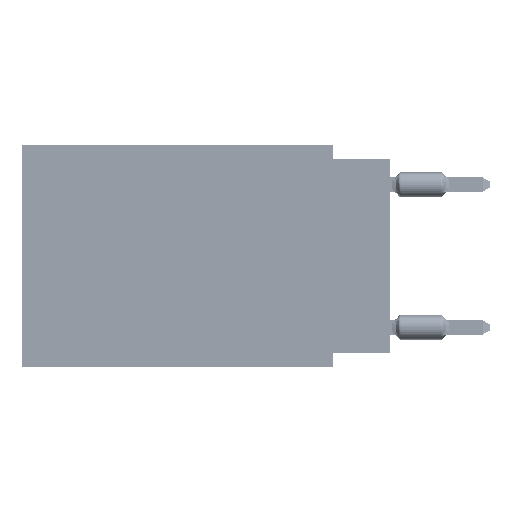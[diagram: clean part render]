
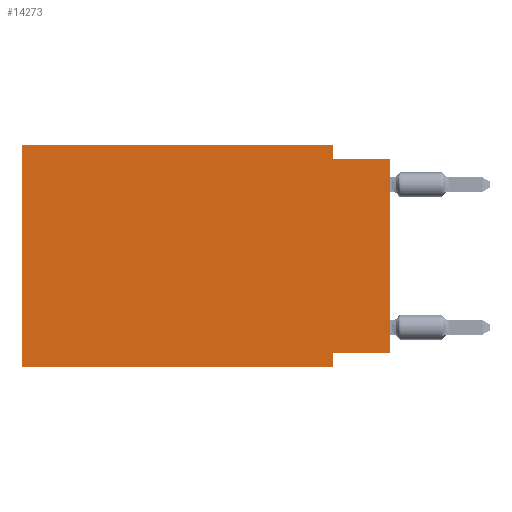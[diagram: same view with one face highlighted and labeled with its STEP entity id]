
A CAD part, left-side view. The second image highlights one B-rep face of the part: STEP entity #14273.
In plain terms, the highlighted planar face has unit normal (-1, 0, 0).
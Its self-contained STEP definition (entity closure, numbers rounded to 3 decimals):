
#194 = EDGE_CURVE ( 'NONE', #3781, #33344, #15759, .T. ) ;
#601 = CARTESIAN_POINT ( 'NONE',  ( 0., 0., -9.271 ) ) ;
#1645 = DIRECTION ( 'NONE',  ( 0., 0., 1. ) ) ;
#1699 = LINE ( 'NONE', #14349, #16346 ) ;
#2934 = ORIENTED_EDGE ( 'NONE', *, *, #26438, .F. ) ;
#3781 = VERTEX_POINT ( 'NONE', #601 ) ;
#3854 = VECTOR ( 'NONE', #1645, 1000. ) ;
#4674 = CARTESIAN_POINT ( 'NONE',  ( 0., 0., -0.635 ) ) ;
#5624 = VERTEX_POINT ( 'NONE', #8807 ) ;
#5972 = DIRECTION ( 'NONE',  ( 0., -1., 0. ) ) ;
#7640 = CARTESIAN_POINT ( 'NONE',  ( 0., 0., 0. ) ) ;
#8581 = DIRECTION ( 'NONE',  ( 0., -1., 0. ) ) ;
#8807 = CARTESIAN_POINT ( 'NONE',  ( 0., 2.54, -0.635 ) ) ;
#9232 = ORIENTED_EDGE ( 'NONE', *, *, #44847, .F. ) ;
#9246 = CARTESIAN_POINT ( 'NONE',  ( 0., 16.383, 0. ) ) ;
#10726 = DIRECTION ( 'NONE',  ( 0., -1., 0. ) ) ;
#11230 = CARTESIAN_POINT ( 'NONE',  ( 0., 2.54, 0. ) ) ;
#11405 = EDGE_CURVE ( 'NONE', #27333, #56095, #11659, .T. ) ;
#11659 = LINE ( 'NONE', #47135, #54206 ) ;
#13464 = EDGE_CURVE ( 'NONE', #56095, #5624, #46716, .T. ) ;
#14273 = ADVANCED_FACE ( 'NONE', ( #47456 ), #15294, .F. ) ;
#14349 = CARTESIAN_POINT ( 'NONE',  ( 0., 16.383, -9.906 ) ) ;
#14377 = CARTESIAN_POINT ( 'NONE',  ( 0., 2.54, -9.906 ) ) ;
#15294 = PLANE ( 'NONE',  #59230 ) ;
#15759 = LINE ( 'NONE', #7640, #3854 ) ;
#16346 = VECTOR ( 'NONE', #10726, 1000. ) ;
#16832 = ORIENTED_EDGE ( 'NONE', *, *, #58958, .F. ) ;
#17105 = ORIENTED_EDGE ( 'NONE', *, *, #44590, .T. ) ;
#19935 = EDGE_CURVE ( 'NONE', #44087, #50458, #32715, .T. ) ;
#23075 = DIRECTION ( 'NONE',  ( 0., 0., 1. ) ) ;
#23708 = CARTESIAN_POINT ( 'NONE',  ( 0., 0., -9.271 ) ) ;
#26438 = EDGE_CURVE ( 'NONE', #3781, #44087, #45647, .T. ) ;
#27333 = VERTEX_POINT ( 'NONE', #48832 ) ;
#27657 = CARTESIAN_POINT ( 'NONE',  ( 0., 2.54, -9.271 ) ) ;
#30799 = ORIENTED_EDGE ( 'NONE', *, *, #11405, .F. ) ;
#31202 = ORIENTED_EDGE ( 'NONE', *, *, #194, .T. ) ;
#32715 = LINE ( 'NONE', #14377, #37526 ) ;
#33344 = VERTEX_POINT ( 'NONE', #53082 ) ;
#33634 = CARTESIAN_POINT ( 'NONE',  ( 0., 16.383, 0. ) ) ;
#34072 = DIRECTION ( 'NONE',  ( 0., 0., -1. ) ) ;
#37526 = VECTOR ( 'NONE', #45943, 1000. ) ;
#37915 = CARTESIAN_POINT ( 'NONE',  ( 0., 16.383, -9.906 ) ) ;
#38467 = EDGE_LOOP ( 'NONE', ( #31202, #9232, #41016, #30799, #16832, #17105, #54673, #2934 ) ) ;
#39680 = CARTESIAN_POINT ( 'NONE',  ( 0., 2.54, 0. ) ) ;
#40014 = VERTEX_POINT ( 'NONE', #37915 ) ;
#41016 = ORIENTED_EDGE ( 'NONE', *, *, #13464, .F. ) ;
#41204 = VECTOR ( 'NONE', #23075, 1000. ) ;
#42294 = LINE ( 'NONE', #9246, #41204 ) ;
#43213 = VECTOR ( 'NONE', #8581, 1000. ) ;
#44087 = VERTEX_POINT ( 'NONE', #27657 ) ;
#44590 = EDGE_CURVE ( 'NONE', #40014, #50458, #1699, .T. ) ;
#44847 = EDGE_CURVE ( 'NONE', #5624, #33344, #53955, .T. ) ;
#45647 = LINE ( 'NONE', #23708, #56006 ) ;
#45943 = DIRECTION ( 'NONE',  ( 0., 0., -1. ) ) ;
#46241 = DIRECTION ( 'NONE',  ( 0., 1., 0. ) ) ;
#46716 = LINE ( 'NONE', #11230, #57311 ) ;
#47135 = CARTESIAN_POINT ( 'NONE',  ( 0., 16.383, 0. ) ) ;
#47456 = FACE_OUTER_BOUND ( 'NONE', #38467, .T. ) ;
#48832 = CARTESIAN_POINT ( 'NONE',  ( 0., 16.383, 0. ) ) ;
#50458 = VERTEX_POINT ( 'NONE', #50782 ) ;
#50782 = CARTESIAN_POINT ( 'NONE',  ( 0., 2.54, -9.906 ) ) ;
#51378 = DIRECTION ( 'NONE',  ( 1., 0., 0. ) ) ;
#51968 = DIRECTION ( 'NONE',  ( 0., 0., -1. ) ) ;
#53082 = CARTESIAN_POINT ( 'NONE',  ( 0., 0., -0.635 ) ) ;
#53955 = LINE ( 'NONE', #4674, #43213 ) ;
#54206 = VECTOR ( 'NONE', #5972, 1000. ) ;
#54673 = ORIENTED_EDGE ( 'NONE', *, *, #19935, .F. ) ;
#56006 = VECTOR ( 'NONE', #46241, 1000. ) ;
#56095 = VERTEX_POINT ( 'NONE', #39680 ) ;
#57311 = VECTOR ( 'NONE', #34072, 1000. ) ;
#58958 = EDGE_CURVE ( 'NONE', #40014, #27333, #42294, .T. ) ;
#59230 = AXIS2_PLACEMENT_3D ( 'NONE', #33634, #51378, #51968 ) ;
